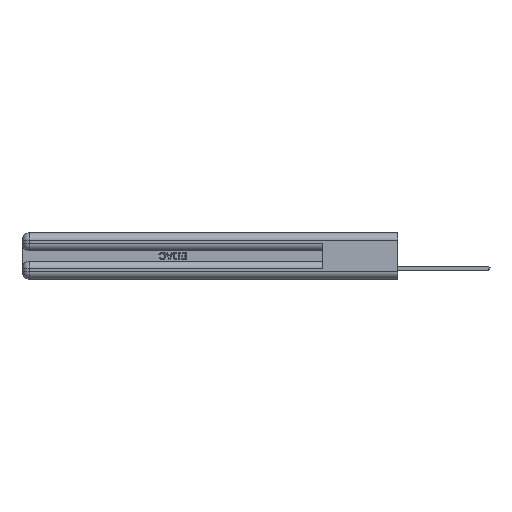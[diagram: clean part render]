
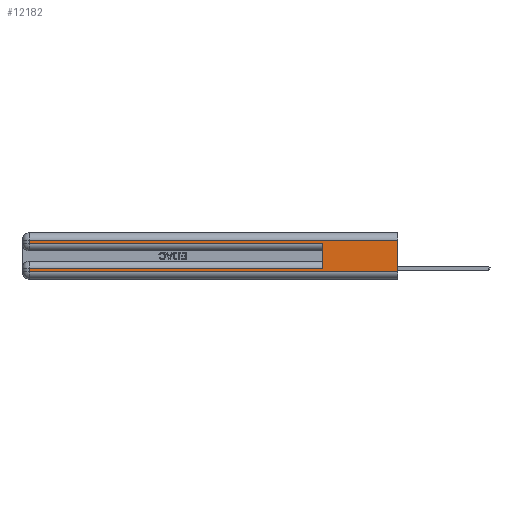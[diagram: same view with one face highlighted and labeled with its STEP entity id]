
A CAD part, left-side view. The second image highlights one B-rep face of the part: STEP entity #12182.
In plain terms, the highlighted planar face has unit normal (-1, 0, 0).
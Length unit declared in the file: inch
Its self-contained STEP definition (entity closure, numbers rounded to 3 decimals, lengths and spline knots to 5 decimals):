
#236 = CARTESIAN_POINT ( 'NONE',  ( 0., 0., 0.085 ) ) ;
#737 = FACE_OUTER_BOUND ( 'NONE', #1101, .T. ) ;
#1101 = EDGE_LOOP ( 'NONE', ( #2109, #40535, #13401, #12092, #38067, #31068, #7686, #28184 ) ) ;
#2109 = ORIENTED_EDGE ( 'NONE', *, *, #19450, .F. ) ;
#2399 = DIRECTION ( 'NONE',  ( 0., 0., 1. ) ) ;
#2788 = CARTESIAN_POINT ( 'NONE',  ( 0., 0., 0.31 ) ) ;
#4545 = VERTEX_POINT ( 'NONE', #8038 ) ;
#6320 = DIRECTION ( 'NONE',  ( 0., 0., -1. ) ) ;
#6409 = CARTESIAN_POINT ( 'NONE',  ( 0., 2.94, 0.37 ) ) ;
#6612 = DIRECTION ( 'NONE',  ( 1., 0., 0. ) ) ;
#6766 = CARTESIAN_POINT ( 'NONE',  ( 0., 0., 0.37 ) ) ;
#6904 = CARTESIAN_POINT ( 'NONE',  ( 0., 0., 0.06 ) ) ;
#7686 = ORIENTED_EDGE ( 'NONE', *, *, #26049, .T. ) ;
#7719 = DIRECTION ( 'NONE',  ( 0., 0., -1. ) ) ;
#7917 = CARTESIAN_POINT ( 'NONE',  ( 0., 0., 0.06 ) ) ;
#8038 = CARTESIAN_POINT ( 'NONE',  ( 0., 0.6, 0.285 ) ) ;
#8837 = VERTEX_POINT ( 'NONE', #40220 ) ;
#11760 = LINE ( 'NONE', #39296, #38512 ) ;
#12073 = VERTEX_POINT ( 'NONE', #29373 ) ;
#12092 = ORIENTED_EDGE ( 'NONE', *, *, #15030, .T. ) ;
#12182 = ADVANCED_FACE ( 'NONE', ( #737 ), #37710, .F. ) ;
#12459 = VECTOR ( 'NONE', #21581, 39.37008 ) ;
#12770 = VERTEX_POINT ( 'NONE', #42764 ) ;
#13401 = ORIENTED_EDGE ( 'NONE', *, *, #17257, .T. ) ;
#14847 = VERTEX_POINT ( 'NONE', #38388 ) ;
#15030 = EDGE_CURVE ( 'NONE', #14847, #4545, #24958, .T. ) ;
#15915 = LINE ( 'NONE', #28861, #42648 ) ;
#16013 = CARTESIAN_POINT ( 'NONE',  ( 0., 0.6, 0.145 ) ) ;
#16618 = LINE ( 'NONE', #30539, #38433 ) ;
#17257 = EDGE_CURVE ( 'NONE', #8837, #14847, #11760, .T. ) ;
#17791 = EDGE_CURVE ( 'NONE', #19170, #25963, #33838, .T. ) ;
#19170 = VERTEX_POINT ( 'NONE', #29818 ) ;
#19450 = EDGE_CURVE ( 'NONE', #37351, #25963, #15915, .T. ) ;
#21300 = EDGE_CURVE ( 'NONE', #12770, #12073, #44124, .T. ) ;
#21581 = DIRECTION ( 'NONE',  ( 0., -1., 0. ) ) ;
#22627 = LINE ( 'NONE', #6409, #37921 ) ;
#23451 = VECTOR ( 'NONE', #42275, 39.37008 ) ;
#24958 = LINE ( 'NONE', #35909, #12459 ) ;
#25963 = VERTEX_POINT ( 'NONE', #6904 ) ;
#26049 = EDGE_CURVE ( 'NONE', #12073, #19170, #22627, .T. ) ;
#28184 = ORIENTED_EDGE ( 'NONE', *, *, #17791, .T. ) ;
#28861 = CARTESIAN_POINT ( 'NONE',  ( 0., 0., 0.37 ) ) ;
#29373 = CARTESIAN_POINT ( 'NONE',  ( 0., 2.94, 0.085 ) ) ;
#29818 = CARTESIAN_POINT ( 'NONE',  ( 0., 2.94, 0.06 ) ) ;
#30539 = CARTESIAN_POINT ( 'NONE',  ( 0., 0., 0.31 ) ) ;
#30618 = LINE ( 'NONE', #16013, #35026 ) ;
#31068 = ORIENTED_EDGE ( 'NONE', *, *, #21300, .T. ) ;
#31347 = DIRECTION ( 'NONE',  ( 0., 1., 0. ) ) ;
#32413 = DIRECTION ( 'NONE',  ( 0., 0., -1. ) ) ;
#33838 = LINE ( 'NONE', #7917, #23451 ) ;
#35026 = VECTOR ( 'NONE', #2399, 39.37008 ) ;
#35909 = CARTESIAN_POINT ( 'NONE',  ( 0., 0., 0.285 ) ) ;
#37351 = VERTEX_POINT ( 'NONE', #2788 ) ;
#37710 = PLANE ( 'NONE',  #42334 ) ;
#37921 = VECTOR ( 'NONE', #44879, 39.37008 ) ;
#38067 = ORIENTED_EDGE ( 'NONE', *, *, #38423, .F. ) ;
#38388 = CARTESIAN_POINT ( 'NONE',  ( 0., 2.94, 0.285 ) ) ;
#38423 = EDGE_CURVE ( 'NONE', #12770, #4545, #30618, .T. ) ;
#38433 = VECTOR ( 'NONE', #44943, 39.37008 ) ;
#38512 = VECTOR ( 'NONE', #7719, 39.37008 ) ;
#39296 = CARTESIAN_POINT ( 'NONE',  ( 0., 2.94, 0.37 ) ) ;
#40220 = CARTESIAN_POINT ( 'NONE',  ( 0., 2.94, 0.31 ) ) ;
#40535 = ORIENTED_EDGE ( 'NONE', *, *, #42776, .T. ) ;
#41918 = VECTOR ( 'NONE', #31347, 39.37008 ) ;
#42275 = DIRECTION ( 'NONE',  ( 0., -1., 0. ) ) ;
#42334 = AXIS2_PLACEMENT_3D ( 'NONE', #6766, #6612, #6320 ) ;
#42648 = VECTOR ( 'NONE', #32413, 39.37008 ) ;
#42764 = CARTESIAN_POINT ( 'NONE',  ( 0., 0.6, 0.085 ) ) ;
#42776 = EDGE_CURVE ( 'NONE', #37351, #8837, #16618, .T. ) ;
#44124 = LINE ( 'NONE', #236, #41918 ) ;
#44879 = DIRECTION ( 'NONE',  ( 0., 0., -1. ) ) ;
#44943 = DIRECTION ( 'NONE',  ( 0., 1., 0. ) ) ;
